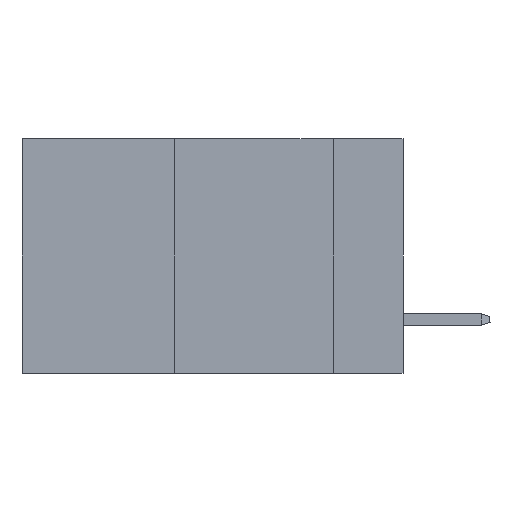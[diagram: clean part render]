
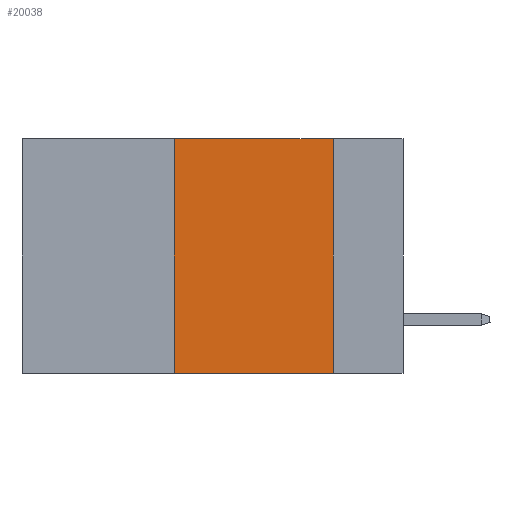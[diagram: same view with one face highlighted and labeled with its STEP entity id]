
A CAD part, left-side view. The second image highlights one B-rep face of the part: STEP entity #20038.
In plain terms, the highlighted planar face has unit normal (-1, 0, 0).
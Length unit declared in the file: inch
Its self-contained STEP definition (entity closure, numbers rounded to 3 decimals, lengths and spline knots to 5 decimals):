
#307 = LINE ( 'NONE', #18155, #11382 ) ;
#1468 = CARTESIAN_POINT ( 'NONE',  ( 0., 0.11, 0. ) ) ;
#2715 = DIRECTION ( 'NONE',  ( 0., -1., 0. ) ) ;
#3132 = VERTEX_POINT ( 'NONE', #10201 ) ;
#3758 = AXIS2_PLACEMENT_3D ( 'NONE', #7810, #25005, #12141 ) ;
#4676 = ORIENTED_EDGE ( 'NONE', *, *, #28926, .F. ) ;
#6412 = VERTEX_POINT ( 'NONE', #16816 ) ;
#7810 = CARTESIAN_POINT ( 'NONE',  ( 0., 0.6, 0. ) ) ;
#7916 = LINE ( 'NONE', #30614, #24141 ) ;
#9428 = ORIENTED_EDGE ( 'NONE', *, *, #25868, .T. ) ;
#10201 = CARTESIAN_POINT ( 'NONE',  ( 0., 0.36, -0.37 ) ) ;
#10487 = DIRECTION ( 'NONE',  ( 0., 0., 1. ) ) ;
#11101 = LINE ( 'NONE', #21298, #11831 ) ;
#11382 = VECTOR ( 'NONE', #10487, 39.37008 ) ;
#11831 = VECTOR ( 'NONE', #31330, 39.37008 ) ;
#12141 = DIRECTION ( 'NONE',  ( 0., 0., -1. ) ) ;
#13595 = VECTOR ( 'NONE', #17088, 39.37008 ) ;
#16421 = EDGE_LOOP ( 'NONE', ( #4676, #29170, #16540, #9428 ) ) ;
#16540 = ORIENTED_EDGE ( 'NONE', *, *, #26910, .F. ) ;
#16552 = VERTEX_POINT ( 'NONE', #19124 ) ;
#16816 = CARTESIAN_POINT ( 'NONE',  ( 0., 0.11, -0.37 ) ) ;
#17088 = DIRECTION ( 'NONE',  ( 0., 0., -1. ) ) ;
#18155 = CARTESIAN_POINT ( 'NONE',  ( 0., 0.36, 0. ) ) ;
#19124 = CARTESIAN_POINT ( 'NONE',  ( 0., 0.36, 0. ) ) ;
#19610 = LINE ( 'NONE', #29806, #13595 ) ;
#20038 = ADVANCED_FACE ( 'NONE', ( #27514 ), #28173, .F. ) ;
#21298 = CARTESIAN_POINT ( 'NONE',  ( 0., 0.6, 0. ) ) ;
#24141 = VECTOR ( 'NONE', #2715, 39.37008 ) ;
#25005 = DIRECTION ( 'NONE',  ( 1., 0., 0. ) ) ;
#25568 = EDGE_CURVE ( 'NONE', #16552, #32543, #11101, .T. ) ;
#25868 = EDGE_CURVE ( 'NONE', #3132, #6412, #7916, .T. ) ;
#26910 = EDGE_CURVE ( 'NONE', #3132, #16552, #307, .T. ) ;
#27514 = FACE_OUTER_BOUND ( 'NONE', #16421, .T. ) ;
#28173 = PLANE ( 'NONE',  #3758 ) ;
#28926 = EDGE_CURVE ( 'NONE', #32543, #6412, #19610, .T. ) ;
#29170 = ORIENTED_EDGE ( 'NONE', *, *, #25568, .F. ) ;
#29806 = CARTESIAN_POINT ( 'NONE',  ( 0., 0.11, 0. ) ) ;
#30614 = CARTESIAN_POINT ( 'NONE',  ( 0., 0.6, -0.37 ) ) ;
#31330 = DIRECTION ( 'NONE',  ( 0., -1., 0. ) ) ;
#32543 = VERTEX_POINT ( 'NONE', #1468 ) ;
